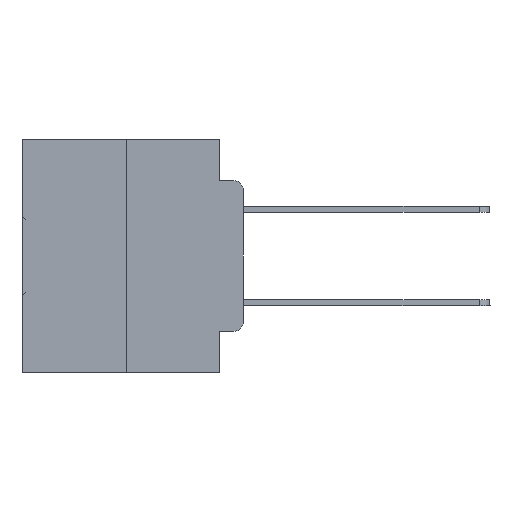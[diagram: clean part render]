
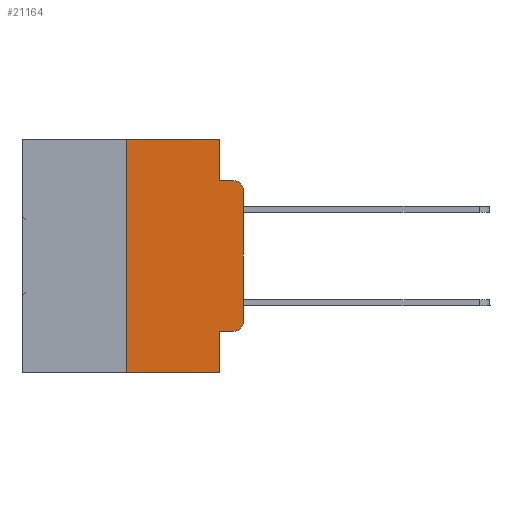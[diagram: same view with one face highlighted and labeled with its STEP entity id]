
A CAD part, left-side view. The second image highlights one B-rep face of the part: STEP entity #21164.
In plain terms, the highlighted planar face has unit normal (-1, 0, 0).
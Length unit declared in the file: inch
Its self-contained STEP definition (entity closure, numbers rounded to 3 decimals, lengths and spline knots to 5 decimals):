
#47 = VERTEX_POINT ( 'NONE', #27807 ) ;
#175 = VERTEX_POINT ( 'NONE', #31101 ) ;
#589 = CARTESIAN_POINT ( 'NONE',  ( 0., 0.051, -0.0885 ) ) ;
#746 = CARTESIAN_POINT ( 'NONE',  ( 0., 0.25, -0.5 ) ) ;
#1858 = VERTEX_POINT ( 'NONE', #12814 ) ;
#2345 = CARTESIAN_POINT ( 'NONE',  ( 0., 0.051, 0. ) ) ;
#2766 = EDGE_CURVE ( 'NONE', #8489, #5863, #5883, .T. ) ;
#3205 = CIRCLE ( 'NONE', #28689, 0.02 ) ;
#3300 = CARTESIAN_POINT ( 'NONE',  ( 0., 0., -0.1085 ) ) ;
#4925 = DIRECTION ( 'NONE',  ( 0., 0., -1. ) ) ;
#5263 = VECTOR ( 'NONE', #23337, 39.37008 ) ;
#5472 = DIRECTION ( 'NONE',  ( 0., -1., 0. ) ) ;
#5550 = LINE ( 'NONE', #16443, #26225 ) ;
#5863 = VERTEX_POINT ( 'NONE', #30173 ) ;
#5883 = CIRCLE ( 'NONE', #22475, 0.02 ) ;
#7386 = CARTESIAN_POINT ( 'NONE',  ( 0., 0.473, 0. ) ) ;
#7682 = FACE_OUTER_BOUND ( 'NONE', #19733, .T. ) ;
#8489 = VERTEX_POINT ( 'NONE', #23257 ) ;
#8908 = CARTESIAN_POINT ( 'NONE',  ( 0., 0.02, -0.1085 ) ) ;
#8942 = ORIENTED_EDGE ( 'NONE', *, *, #24773, .F. ) ;
#9602 = VECTOR ( 'NONE', #10137, 39.37008 ) ;
#10137 = DIRECTION ( 'NONE',  ( 0., 0., 1. ) ) ;
#11047 = CARTESIAN_POINT ( 'NONE',  ( 0., 0.25, 0. ) ) ;
#12412 = LINE ( 'NONE', #33939, #9602 ) ;
#12749 = CARTESIAN_POINT ( 'NONE',  ( 0., 0.02, -0.3915 ) ) ;
#12814 = CARTESIAN_POINT ( 'NONE',  ( 0., 0.051, -0.4115 ) ) ;
#13326 = ORIENTED_EDGE ( 'NONE', *, *, #22481, .F. ) ;
#13387 = LINE ( 'NONE', #32308, #14150 ) ;
#13500 = EDGE_CURVE ( 'NONE', #47, #32524, #20458, .T. ) ;
#13559 = LINE ( 'NONE', #589, #21782 ) ;
#13681 = VECTOR ( 'NONE', #32079, 39.37008 ) ;
#14150 = VECTOR ( 'NONE', #24161, 39.37008 ) ;
#15266 = ORIENTED_EDGE ( 'NONE', *, *, #13500, .F. ) ;
#15586 = EDGE_CURVE ( 'NONE', #5863, #22189, #23903, .T. ) ;
#15983 = CARTESIAN_POINT ( 'NONE',  ( 0., 0.051, -0.5 ) ) ;
#16443 = CARTESIAN_POINT ( 'NONE',  ( 0., 0.473, -0.5 ) ) ;
#18038 = ORIENTED_EDGE ( 'NONE', *, *, #2766, .T. ) ;
#18222 = CARTESIAN_POINT ( 'NONE',  ( 0., 0.473, 0. ) ) ;
#18697 = DIRECTION ( 'NONE',  ( 0., -1., 0. ) ) ;
#19217 = AXIS2_PLACEMENT_3D ( 'NONE', #18222, #28665, #4925 ) ;
#19733 = EDGE_LOOP ( 'NONE', ( #28898, #19929, #31885, #15266, #8942, #13326, #23869, #25281, #27948, #18038 ) ) ;
#19928 = VERTEX_POINT ( 'NONE', #11047 ) ;
#19929 = ORIENTED_EDGE ( 'NONE', *, *, #27640, .T. ) ;
#20458 = LINE ( 'NONE', #33659, #34104 ) ;
#20526 = LINE ( 'NONE', #2345, #25770 ) ;
#21164 = ADVANCED_FACE ( 'NONE', ( #7682 ), #28986, .F. ) ;
#21782 = VECTOR ( 'NONE', #5472, 39.37008 ) ;
#22189 = VERTEX_POINT ( 'NONE', #3300 ) ;
#22218 = EDGE_CURVE ( 'NONE', #32751, #26644, #5550, .T. ) ;
#22475 = AXIS2_PLACEMENT_3D ( 'NONE', #12749, #33401, #25595 ) ;
#22481 = EDGE_CURVE ( 'NONE', #32751, #19928, #12412, .T. ) ;
#23257 = CARTESIAN_POINT ( 'NONE',  ( 0., 0.02, -0.4115 ) ) ;
#23337 = DIRECTION ( 'NONE',  ( 0., -1., 0. ) ) ;
#23506 = LINE ( 'NONE', #7386, #5263 ) ;
#23748 = CARTESIAN_POINT ( 'NONE',  ( 0., 0., 0. ) ) ;
#23760 = EDGE_CURVE ( 'NONE', #1858, #26644, #20526, .T. ) ;
#23869 = ORIENTED_EDGE ( 'NONE', *, *, #22218, .T. ) ;
#23903 = LINE ( 'NONE', #23748, #13681 ) ;
#24161 = DIRECTION ( 'NONE',  ( 0., -1., 0. ) ) ;
#24773 = EDGE_CURVE ( 'NONE', #19928, #47, #23506, .T. ) ;
#25281 = ORIENTED_EDGE ( 'NONE', *, *, #23760, .F. ) ;
#25595 = DIRECTION ( 'NONE',  ( 0., 0., -1. ) ) ;
#25770 = VECTOR ( 'NONE', #31293, 39.37008 ) ;
#26225 = VECTOR ( 'NONE', #18697, 39.37008 ) ;
#26644 = VERTEX_POINT ( 'NONE', #15983 ) ;
#27189 = CARTESIAN_POINT ( 'NONE',  ( 0., 0.051, -0.0885 ) ) ;
#27640 = EDGE_CURVE ( 'NONE', #22189, #175, #3205, .T. ) ;
#27807 = CARTESIAN_POINT ( 'NONE',  ( 0., 0.051, 0. ) ) ;
#27948 = ORIENTED_EDGE ( 'NONE', *, *, #32799, .T. ) ;
#28665 = DIRECTION ( 'NONE',  ( 1., 0., 0. ) ) ;
#28689 = AXIS2_PLACEMENT_3D ( 'NONE', #8908, #30272, #30442 ) ;
#28898 = ORIENTED_EDGE ( 'NONE', *, *, #15586, .T. ) ;
#28986 = PLANE ( 'NONE',  #19217 ) ;
#29397 = EDGE_CURVE ( 'NONE', #32524, #175, #13559, .T. ) ;
#30173 = CARTESIAN_POINT ( 'NONE',  ( 0., 0., -0.3915 ) ) ;
#30272 = DIRECTION ( 'NONE',  ( -1., 0., 0. ) ) ;
#30442 = DIRECTION ( 'NONE',  ( 0., 0., -1. ) ) ;
#31057 = DIRECTION ( 'NONE',  ( 0., 0., -1. ) ) ;
#31101 = CARTESIAN_POINT ( 'NONE',  ( 0., 0.02, -0.0885 ) ) ;
#31293 = DIRECTION ( 'NONE',  ( 0., 0., -1. ) ) ;
#31885 = ORIENTED_EDGE ( 'NONE', *, *, #29397, .F. ) ;
#32079 = DIRECTION ( 'NONE',  ( 0., 0., 1. ) ) ;
#32308 = CARTESIAN_POINT ( 'NONE',  ( 0., 0.051, -0.4115 ) ) ;
#32524 = VERTEX_POINT ( 'NONE', #27189 ) ;
#32751 = VERTEX_POINT ( 'NONE', #746 ) ;
#32799 = EDGE_CURVE ( 'NONE', #1858, #8489, #13387, .T. ) ;
#33401 = DIRECTION ( 'NONE',  ( -1., 0., 0. ) ) ;
#33659 = CARTESIAN_POINT ( 'NONE',  ( 0., 0.051, 0. ) ) ;
#33939 = CARTESIAN_POINT ( 'NONE',  ( 0., 0.25, 0. ) ) ;
#34104 = VECTOR ( 'NONE', #31057, 39.37008 ) ;
